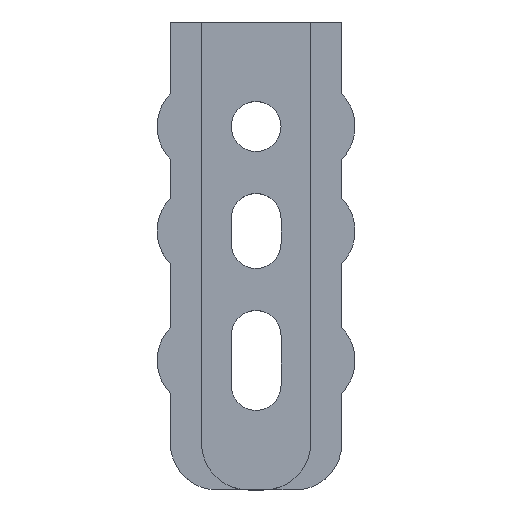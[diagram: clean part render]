
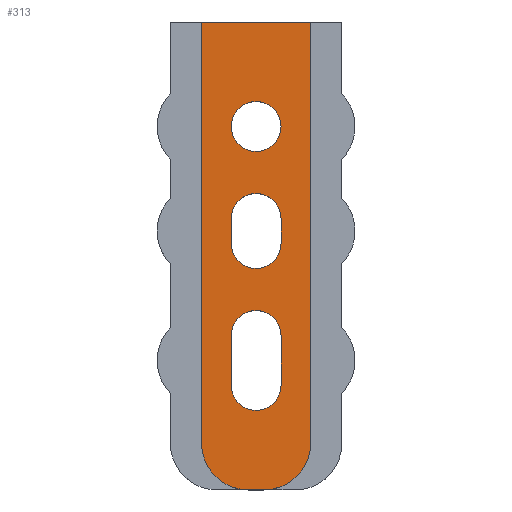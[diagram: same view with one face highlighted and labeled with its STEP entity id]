
A CAD part, top view. The second image highlights one B-rep face of the part: STEP entity #313.
In plain terms, the highlighted planar face has unit normal (0, 0, 1).
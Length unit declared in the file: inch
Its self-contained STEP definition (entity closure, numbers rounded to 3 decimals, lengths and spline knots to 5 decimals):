
#4 = ORIENTED_EDGE ( 'NONE', *, *, #841, .F. ) ;
#8 = DIRECTION ( 'NONE',  ( 0., 0., -1. ) ) ;
#11 = FACE_BOUND ( 'NONE', #1175, .T. ) ;
#15 = AXIS2_PLACEMENT_3D ( 'NONE', #998, #1486, #279 ) ;
#20 = CARTESIAN_POINT ( 'NONE',  ( -0.0335, 0.083, 0.0175 ) ) ;
#32 = VERTEX_POINT ( 'NONE', #754 ) ;
#37 = DIRECTION ( 'NONE',  ( 1., 0., 0. ) ) ;
#42 = CARTESIAN_POINT ( 'NONE',  ( 0.005, -0.12, 0.0175 ) ) ;
#48 = CARTESIAN_POINT ( 'NONE',  ( 0., 0.008, 0.0175 ) ) ;
#56 = CARTESIAN_POINT ( 'NONE',  ( 0., 0.024, 0.0175 ) ) ;
#63 = VERTEX_POINT ( 'NONE', #1124 ) ;
#71 = DIRECTION ( 'NONE',  ( 1., 0., 0. ) ) ;
#78 = VERTEX_POINT ( 'NONE', #1475 ) ;
#79 = AXIS2_PLACEMENT_3D ( 'NONE', #48, #527, #71 ) ;
#82 = CARTESIAN_POINT ( 'NONE',  ( -0.016, -0.083, 0.0175 ) ) ;
#87 = AXIS2_PLACEMENT_3D ( 'NONE', #56, #1515, #1250 ) ;
#89 = ORIENTED_EDGE ( 'NONE', *, *, #494, .F. ) ;
#94 = CIRCLE ( 'NONE', #1299, 0.03 ) ;
#99 = CARTESIAN_POINT ( 'NONE',  ( -0.005, -0.15, 0.0175 ) ) ;
#112 = DIRECTION ( 'NONE',  ( 0., 0., 1. ) ) ;
#118 = VERTEX_POINT ( 'NONE', #1489 ) ;
#121 = DIRECTION ( 'NONE',  ( 0., 0., 1. ) ) ;
#132 = CARTESIAN_POINT ( 'NONE',  ( 0.016, -0.083, 0.0175 ) ) ;
#176 = CIRCLE ( 'NONE', #1261, 0.016 ) ;
#214 = EDGE_CURVE ( 'NONE', #32, #1183, #1505, .T. ) ;
#218 = EDGE_CURVE ( 'NONE', #1144, #452, #436, .T. ) ;
#223 = VECTOR ( 'NONE', #701, 39.37008 ) ;
#224 = ORIENTED_EDGE ( 'NONE', *, *, #214, .F. ) ;
#230 = CARTESIAN_POINT ( 'NONE',  ( -0.016, 0.083, 0.0175 ) ) ;
#241 = CARTESIAN_POINT ( 'NONE',  ( 0.035, -0.15, 0.0175 ) ) ;
#252 = CARTESIAN_POINT ( 'NONE',  ( -0.035, -0.12, 0.0175 ) ) ;
#279 = DIRECTION ( 'NONE',  ( 1., 0., 0. ) ) ;
#288 = CIRCLE ( 'NONE', #1527, 0.016 ) ;
#303 = AXIS2_PLACEMENT_3D ( 'NONE', #1058, #121, #1187 ) ;
#313 = ADVANCED_FACE ( 'NONE', ( #1184, #1198, #835, #11 ), #577, .T. ) ;
#323 = DIRECTION ( 'NONE',  ( -1., 0., 0. ) ) ;
#340 = CARTESIAN_POINT ( 'NONE',  ( -0.016, 0.008, 0.0175 ) ) ;
#362 = LINE ( 'NONE', #241, #1279 ) ;
#378 = LINE ( 'NONE', #612, #437 ) ;
#404 = VECTOR ( 'NONE', #658, 39.37008 ) ;
#407 = LINE ( 'NONE', #1027, #404 ) ;
#411 = CARTESIAN_POINT ( 'NONE',  ( -0.055, 0.15, 0.0175 ) ) ;
#421 = ORIENTED_EDGE ( 'NONE', *, *, #805, .F. ) ;
#428 = EDGE_CURVE ( 'NONE', #979, #452, #568, .T. ) ;
#429 = EDGE_CURVE ( 'NONE', #78, #1144, #362, .T. ) ;
#433 = EDGE_LOOP ( 'NONE', ( #1262, #4 ) ) ;
#436 = LINE ( 'NONE', #411, #1384 ) ;
#437 = VECTOR ( 'NONE', #1361, 39.37008 ) ;
#452 = VERTEX_POINT ( 'NONE', #1364 ) ;
#468 = ORIENTED_EDGE ( 'NONE', *, *, #1107, .F. ) ;
#469 = VERTEX_POINT ( 'NONE', #132 ) ;
#493 = CARTESIAN_POINT ( 'NONE',  ( 0.016, 0.083, 0.0175 ) ) ;
#494 = EDGE_CURVE ( 'NONE', #505, #1154, #744, .T. ) ;
#499 = CARTESIAN_POINT ( 'NONE',  ( 0., -0.051, 0.0175 ) ) ;
#504 = DIRECTION ( 'NONE',  ( -1., 0., 0. ) ) ;
#505 = VERTEX_POINT ( 'NONE', #608 ) ;
#527 = DIRECTION ( 'NONE',  ( 0., 0., 1. ) ) ;
#537 = ORIENTED_EDGE ( 'NONE', *, *, #428, .F. ) ;
#542 = DIRECTION ( 'NONE',  ( 1., 0., 0. ) ) ;
#568 = LINE ( 'NONE', #1452, #223 ) ;
#569 = VERTEX_POINT ( 'NONE', #493 ) ;
#572 = DIRECTION ( 'NONE',  ( 1., 0., 0. ) ) ;
#577 = PLANE ( 'NONE',  #1507 ) ;
#598 = VECTOR ( 'NONE', #620, 39.37008 ) ;
#608 = CARTESIAN_POINT ( 'NONE',  ( -0.016, -0.051, 0.0175 ) ) ;
#612 = CARTESIAN_POINT ( 'NONE',  ( -0.016, 0.008, 0.0175 ) ) ;
#620 = DIRECTION ( 'NONE',  ( 0., -1., 0. ) ) ;
#658 = DIRECTION ( 'NONE',  ( 0., 1., 0. ) ) ;
#701 = DIRECTION ( 'NONE',  ( 0., 1., 0. ) ) ;
#708 = EDGE_CURVE ( 'NONE', #1183, #63, #1089, .T. ) ;
#722 = EDGE_CURVE ( 'NONE', #469, #1517, #407, .T. ) ;
#744 = LINE ( 'NONE', #1109, #598 ) ;
#754 = CARTESIAN_POINT ( 'NONE',  ( 0.016, 0.008, 0.0175 ) ) ;
#781 = CIRCLE ( 'NONE', #1474, 0.03 ) ;
#805 = EDGE_CURVE ( 'NONE', #1162, #979, #781, .T. ) ;
#814 = VERTEX_POINT ( 'NONE', #230 ) ;
#819 = ORIENTED_EDGE ( 'NONE', *, *, #722, .F. ) ;
#822 = ORIENTED_EDGE ( 'NONE', *, *, #429, .T. ) ;
#825 = DIRECTION ( 'NONE',  ( 1., 0., 0. ) ) ;
#828 = EDGE_CURVE ( 'NONE', #1154, #469, #861, .T. ) ;
#830 = CARTESIAN_POINT ( 'NONE',  ( 0., 0.083, 0.0175 ) ) ;
#835 = FACE_BOUND ( 'NONE', #1150, .T. ) ;
#838 = DIRECTION ( 'NONE',  ( 1., 0., 0. ) ) ;
#841 = EDGE_CURVE ( 'NONE', #569, #814, #176, .T. ) ;
#861 = CIRCLE ( 'NONE', #303, 0.016 ) ;
#865 = DIRECTION ( 'NONE',  ( 0., 1., 0. ) ) ;
#931 = DIRECTION ( 'NONE',  ( 0., 0., 1. ) ) ;
#957 = VECTOR ( 'NONE', #1158, 39.37008 ) ;
#967 = ORIENTED_EDGE ( 'NONE', *, *, #1131, .F. ) ;
#979 = VERTEX_POINT ( 'NONE', #252 ) ;
#997 = CIRCLE ( 'NONE', #15, 0.016 ) ;
#998 = CARTESIAN_POINT ( 'NONE',  ( 0., 0.083, 0.0175 ) ) ;
#1027 = CARTESIAN_POINT ( 'NONE',  ( 0.016, -0.083, 0.0175 ) ) ;
#1056 = ORIENTED_EDGE ( 'NONE', *, *, #708, .F. ) ;
#1058 = CARTESIAN_POINT ( 'NONE',  ( 0., -0.083, 0.0175 ) ) ;
#1085 = EDGE_CURVE ( 'NONE', #63, #1178, #378, .T. ) ;
#1089 = CIRCLE ( 'NONE', #87, 0.016 ) ;
#1107 = EDGE_CURVE ( 'NONE', #78, #118, #94, .T. ) ;
#1109 = CARTESIAN_POINT ( 'NONE',  ( -0.016, -0.083, 0.0175 ) ) ;
#1124 = CARTESIAN_POINT ( 'NONE',  ( -0.016, 0.024, 0.0175 ) ) ;
#1131 = EDGE_CURVE ( 'NONE', #1517, #505, #288, .T. ) ;
#1144 = VERTEX_POINT ( 'NONE', #1229 ) ;
#1150 = EDGE_LOOP ( 'NONE', ( #224, #1380, #1315, #1056 ) ) ;
#1154 = VERTEX_POINT ( 'NONE', #82 ) ;
#1158 = DIRECTION ( 'NONE',  ( 0., 1., 0. ) ) ;
#1162 = VERTEX_POINT ( 'NONE', #99 ) ;
#1175 = EDGE_LOOP ( 'NONE', ( #819, #1333, #89, #967 ) ) ;
#1178 = VERTEX_POINT ( 'NONE', #340 ) ;
#1183 = VERTEX_POINT ( 'NONE', #1420 ) ;
#1184 = FACE_OUTER_BOUND ( 'NONE', #1193, .T. ) ;
#1187 = DIRECTION ( 'NONE',  ( 1., 0., 0. ) ) ;
#1189 = ORIENTED_EDGE ( 'NONE', *, *, #1502, .T. ) ;
#1193 = EDGE_LOOP ( 'NONE', ( #421, #1189, #468, #822, #1216, #537 ) ) ;
#1198 = FACE_BOUND ( 'NONE', #433, .T. ) ;
#1216 = ORIENTED_EDGE ( 'NONE', *, *, #218, .T. ) ;
#1223 = DIRECTION ( 'NONE',  ( 0., 0., 1. ) ) ;
#1229 = CARTESIAN_POINT ( 'NONE',  ( 0.035, 0.15, 0.0175 ) ) ;
#1241 = LINE ( 'NONE', #1257, #1470 ) ;
#1250 = DIRECTION ( 'NONE',  ( 1., 0., 0. ) ) ;
#1256 = CARTESIAN_POINT ( 'NONE',  ( 0.016, 0.008, 0.0175 ) ) ;
#1257 = CARTESIAN_POINT ( 'NONE',  ( -0.025, -0.15, 0.0175 ) ) ;
#1261 = AXIS2_PLACEMENT_3D ( 'NONE', #830, #931, #838 ) ;
#1262 = ORIENTED_EDGE ( 'NONE', *, *, #1445, .F. ) ;
#1279 = VECTOR ( 'NONE', #865, 39.37008 ) ;
#1299 = AXIS2_PLACEMENT_3D ( 'NONE', #42, #1476, #504 ) ;
#1313 = CIRCLE ( 'NONE', #79, 0.016 ) ;
#1315 = ORIENTED_EDGE ( 'NONE', *, *, #1085, .F. ) ;
#1333 = ORIENTED_EDGE ( 'NONE', *, *, #828, .F. ) ;
#1361 = DIRECTION ( 'NONE',  ( 0., -1., 0. ) ) ;
#1364 = CARTESIAN_POINT ( 'NONE',  ( -0.035, 0.15, 0.0175 ) ) ;
#1380 = ORIENTED_EDGE ( 'NONE', *, *, #1458, .F. ) ;
#1384 = VECTOR ( 'NONE', #323, 39.37008 ) ;
#1420 = CARTESIAN_POINT ( 'NONE',  ( 0.016, 0.024, 0.0175 ) ) ;
#1445 = EDGE_CURVE ( 'NONE', #814, #569, #997, .T. ) ;
#1452 = CARTESIAN_POINT ( 'NONE',  ( -0.035, -0.15, 0.0175 ) ) ;
#1458 = EDGE_CURVE ( 'NONE', #1178, #32, #1313, .T. ) ;
#1470 = VECTOR ( 'NONE', #542, 39.37008 ) ;
#1474 = AXIS2_PLACEMENT_3D ( 'NONE', #1545, #8, #572 ) ;
#1475 = CARTESIAN_POINT ( 'NONE',  ( 0.035, -0.12, 0.0175 ) ) ;
#1476 = DIRECTION ( 'NONE',  ( 0., 0., -1. ) ) ;
#1486 = DIRECTION ( 'NONE',  ( 0., 0., 1. ) ) ;
#1488 = CARTESIAN_POINT ( 'NONE',  ( 0.016, -0.051, 0.0175 ) ) ;
#1489 = CARTESIAN_POINT ( 'NONE',  ( 0.005, -0.15, 0.0175 ) ) ;
#1502 = EDGE_CURVE ( 'NONE', #1162, #118, #1241, .T. ) ;
#1505 = LINE ( 'NONE', #1256, #957 ) ;
#1507 = AXIS2_PLACEMENT_3D ( 'NONE', #20, #112, #825 ) ;
#1515 = DIRECTION ( 'NONE',  ( 0., 0., 1. ) ) ;
#1517 = VERTEX_POINT ( 'NONE', #1488 ) ;
#1527 = AXIS2_PLACEMENT_3D ( 'NONE', #499, #1223, #37 ) ;
#1545 = CARTESIAN_POINT ( 'NONE',  ( -0.005, -0.12, 0.0175 ) ) ;
